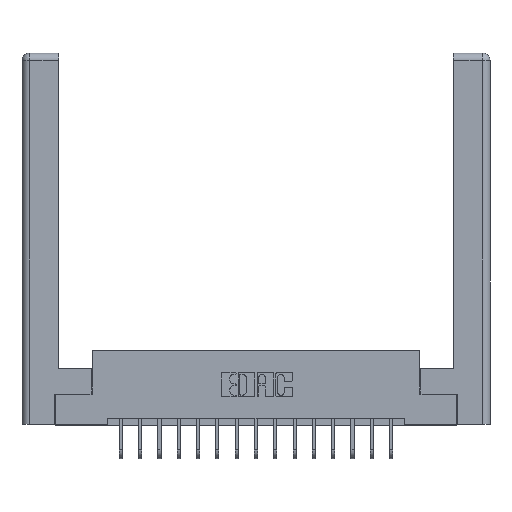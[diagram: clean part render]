
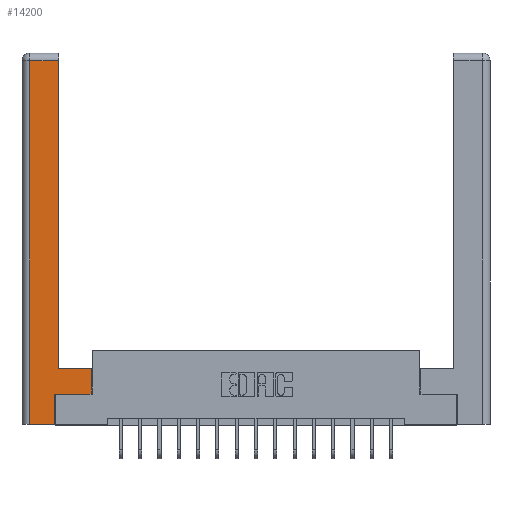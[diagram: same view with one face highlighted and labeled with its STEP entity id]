
A CAD part, top view. The second image highlights one B-rep face of the part: STEP entity #14200.
In plain terms, the highlighted planar face has unit normal (0, 0, 1).
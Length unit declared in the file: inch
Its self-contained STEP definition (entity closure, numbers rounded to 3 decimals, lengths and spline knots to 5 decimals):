
#348 = VERTEX_POINT ( 'NONE', #12098 ) ;
#1476 = CARTESIAN_POINT ( 'NONE',  ( 0.265, 0.245, 0. ) ) ;
#2149 = CARTESIAN_POINT ( 'NONE',  ( 0.295, 0.45, 0. ) ) ;
#2267 = VECTOR ( 'NONE', #17297, 39.37008 ) ;
#2707 = DIRECTION ( 'NONE',  ( 1., 0., 0. ) ) ;
#3192 = CARTESIAN_POINT ( 'NONE',  ( 0.0615, 0., 0. ) ) ;
#3945 = EDGE_CURVE ( 'NONE', #4510, #10459, #16943, .T. ) ;
#4090 = FACE_OUTER_BOUND ( 'NONE', #17606, .T. ) ;
#4113 = ORIENTED_EDGE ( 'NONE', *, *, #15234, .T. ) ;
#4325 = DIRECTION ( 'NONE',  ( 0., 1., 0. ) ) ;
#4346 = CARTESIAN_POINT ( 'NONE',  ( 0.295, 2.94, 0. ) ) ;
#4412 = DIRECTION ( 'NONE',  ( 0., 0., -1. ) ) ;
#4510 = VERTEX_POINT ( 'NONE', #2149 ) ;
#4666 = ORIENTED_EDGE ( 'NONE', *, *, #5324, .T. ) ;
#5055 = LINE ( 'NONE', #7109, #16143 ) ;
#5324 = EDGE_CURVE ( 'NONE', #348, #18916, #7907, .T. ) ;
#5353 = VECTOR ( 'NONE', #18504, 39.37008 ) ;
#5396 = CARTESIAN_POINT ( 'NONE',  ( 0.0615, 0., 0. ) ) ;
#5454 = LINE ( 'NONE', #17173, #6632 ) ;
#5655 = VERTEX_POINT ( 'NONE', #17587 ) ;
#5697 = ORIENTED_EDGE ( 'NONE', *, *, #6399, .T. ) ;
#5880 = ORIENTED_EDGE ( 'NONE', *, *, #18273, .T. ) ;
#6095 = CARTESIAN_POINT ( 'NONE',  ( 0., 0., 0. ) ) ;
#6286 = CARTESIAN_POINT ( 'NONE',  ( 0.295, 3., 0. ) ) ;
#6399 = EDGE_CURVE ( 'NONE', #5655, #348, #5055, .T. ) ;
#6477 = VECTOR ( 'NONE', #7613, 39.37008 ) ;
#6629 = ORIENTED_EDGE ( 'NONE', *, *, #3945, .T. ) ;
#6632 = VECTOR ( 'NONE', #6786, 39.37008 ) ;
#6786 = DIRECTION ( 'NONE',  ( -1., 0., 0. ) ) ;
#7109 = CARTESIAN_POINT ( 'NONE',  ( 0.565, 0.245, 0. ) ) ;
#7541 = CARTESIAN_POINT ( 'NONE',  ( 0.565, 0.45, 0. ) ) ;
#7613 = DIRECTION ( 'NONE',  ( 0., 1., 0. ) ) ;
#7907 = LINE ( 'NONE', #7541, #6477 ) ;
#8066 = CARTESIAN_POINT ( 'NONE',  ( 0.0615, 2.94, 0. ) ) ;
#8192 = CARTESIAN_POINT ( 'NONE',  ( 0.265, 0., 0. ) ) ;
#8719 = LINE ( 'NONE', #17121, #11777 ) ;
#9092 = DIRECTION ( 'NONE',  ( -1., 0., 0. ) ) ;
#9167 = EDGE_CURVE ( 'NONE', #14737, #5655, #18408, .T. ) ;
#9226 = VERTEX_POINT ( 'NONE', #3192 ) ;
#9305 = EDGE_CURVE ( 'NONE', #10459, #16390, #8719, .T. ) ;
#10388 = VECTOR ( 'NONE', #4325, 39.37008 ) ;
#10459 = VERTEX_POINT ( 'NONE', #4346 ) ;
#11535 = EDGE_CURVE ( 'NONE', #16390, #9226, #12899, .T. ) ;
#11660 = ORIENTED_EDGE ( 'NONE', *, *, #9305, .T. ) ;
#11777 = VECTOR ( 'NONE', #14240, 39.37008 ) ;
#11940 = AXIS2_PLACEMENT_3D ( 'NONE', #6095, #4412, #9092 ) ;
#12098 = CARTESIAN_POINT ( 'NONE',  ( 0.565, 0.245, 0. ) ) ;
#12276 = ORIENTED_EDGE ( 'NONE', *, *, #11535, .T. ) ;
#12899 = LINE ( 'NONE', #5396, #2267 ) ;
#13617 = VECTOR ( 'NONE', #15727, 39.37008 ) ;
#14200 = ADVANCED_FACE ( 'NONE', ( #4090 ), #19574, .F. ) ;
#14240 = DIRECTION ( 'NONE',  ( -1., 0., 0. ) ) ;
#14570 = CARTESIAN_POINT ( 'NONE',  ( 0.265, 0., 0. ) ) ;
#14737 = VERTEX_POINT ( 'NONE', #14570 ) ;
#15234 = EDGE_CURVE ( 'NONE', #18916, #4510, #5454, .T. ) ;
#15655 = CARTESIAN_POINT ( 'NONE',  ( 0.565, 0.45, 0. ) ) ;
#15727 = DIRECTION ( 'NONE',  ( 1., 0., 0. ) ) ;
#16143 = VECTOR ( 'NONE', #2707, 39.37008 ) ;
#16197 = LINE ( 'NONE', #8192, #13617 ) ;
#16390 = VERTEX_POINT ( 'NONE', #8066 ) ;
#16943 = LINE ( 'NONE', #6286, #5353 ) ;
#17121 = CARTESIAN_POINT ( 'NONE',  ( 0.0615, 2.94, 0. ) ) ;
#17173 = CARTESIAN_POINT ( 'NONE',  ( 0.295, 0.45, 0. ) ) ;
#17297 = DIRECTION ( 'NONE',  ( 0., -1., 0. ) ) ;
#17587 = CARTESIAN_POINT ( 'NONE',  ( 0.265, 0.245, 0. ) ) ;
#17606 = EDGE_LOOP ( 'NONE', ( #6629, #11660, #12276, #5880, #17869, #5697, #4666, #4113 ) ) ;
#17869 = ORIENTED_EDGE ( 'NONE', *, *, #9167, .T. ) ;
#18273 = EDGE_CURVE ( 'NONE', #9226, #14737, #16197, .T. ) ;
#18408 = LINE ( 'NONE', #1476, #10388 ) ;
#18504 = DIRECTION ( 'NONE',  ( 0., 1., 0. ) ) ;
#18916 = VERTEX_POINT ( 'NONE', #15655 ) ;
#19574 = PLANE ( 'NONE',  #11940 ) ;
